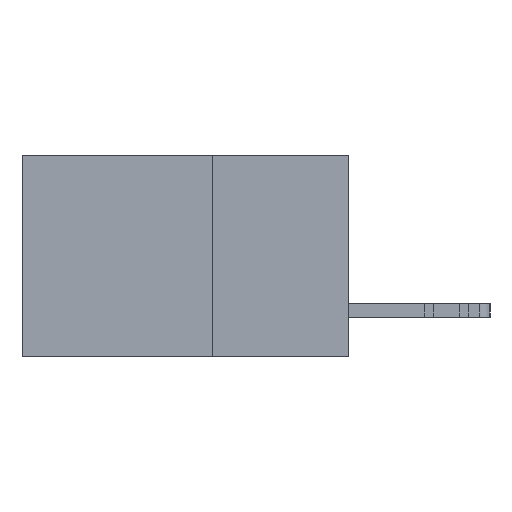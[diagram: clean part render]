
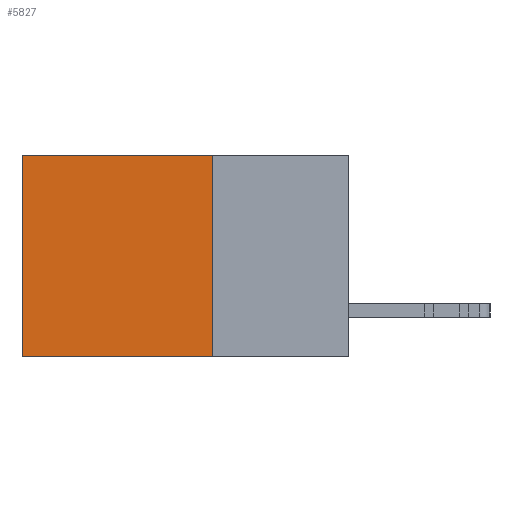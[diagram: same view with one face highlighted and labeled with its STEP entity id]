
A CAD part, left-side view. The second image highlights one B-rep face of the part: STEP entity #5827.
In plain terms, the highlighted planar face has unit normal (-1, 0, 0).
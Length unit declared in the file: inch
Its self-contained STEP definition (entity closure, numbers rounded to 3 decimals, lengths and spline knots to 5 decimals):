
#267 = DIRECTION ( 'NONE',  ( 1., 0., 0. ) ) ;
#484 = VERTEX_POINT ( 'NONE', #6605 ) ;
#1245 = CARTESIAN_POINT ( 'NONE',  ( 0.298, 0.25, -0.37 ) ) ;
#1613 = DIRECTION ( 'NONE',  ( 0., 0., -1. ) ) ;
#3563 = LINE ( 'NONE', #21621, #25673 ) ;
#3666 = EDGE_CURVE ( 'NONE', #4338, #14736, #26336, .T. ) ;
#3944 = DIRECTION ( 'NONE',  ( 0., 0., -1. ) ) ;
#4338 = VERTEX_POINT ( 'NONE', #23929 ) ;
#4529 = VECTOR ( 'NONE', #13940, 39.37008 ) ;
#5827 = ADVANCED_FACE ( 'NONE', ( #6676 ), #24602, .F. ) ;
#6118 = EDGE_CURVE ( 'NONE', #14736, #484, #27677, .T. ) ;
#6283 = EDGE_CURVE ( 'NONE', #4338, #20408, #28006, .T. ) ;
#6605 = CARTESIAN_POINT ( 'NONE',  ( 0.298, 0.6, -0.37 ) ) ;
#6676 = FACE_OUTER_BOUND ( 'NONE', #10706, .T. ) ;
#6752 = CARTESIAN_POINT ( 'NONE',  ( 0.298, 0.25, 0. ) ) ;
#10082 = ORIENTED_EDGE ( 'NONE', *, *, #6118, .F. ) ;
#10706 = EDGE_LOOP ( 'NONE', ( #10852, #10082, #19434, #26820 ) ) ;
#10852 = ORIENTED_EDGE ( 'NONE', *, *, #11824, .T. ) ;
#11417 = CARTESIAN_POINT ( 'NONE',  ( 0.298, 0.25, 0. ) ) ;
#11824 = EDGE_CURVE ( 'NONE', #20408, #484, #3563, .T. ) ;
#13940 = DIRECTION ( 'NONE',  ( 0., 1., 0. ) ) ;
#14221 = CARTESIAN_POINT ( 'NONE',  ( 0.298, 0.6, 0. ) ) ;
#14736 = VERTEX_POINT ( 'NONE', #19982 ) ;
#15842 = DIRECTION ( 'NONE',  ( 0., 0., -1. ) ) ;
#16034 = VECTOR ( 'NONE', #3944, 39.37008 ) ;
#16340 = AXIS2_PLACEMENT_3D ( 'NONE', #11417, #267, #15842 ) ;
#19434 = ORIENTED_EDGE ( 'NONE', *, *, #3666, .F. ) ;
#19982 = CARTESIAN_POINT ( 'NONE',  ( 0.298, 0.25, -0.37 ) ) ;
#20408 = VERTEX_POINT ( 'NONE', #14221 ) ;
#21621 = CARTESIAN_POINT ( 'NONE',  ( 0.298, 0.6, 0. ) ) ;
#23861 = CARTESIAN_POINT ( 'NONE',  ( 0.298, 0.25, 0. ) ) ;
#23929 = CARTESIAN_POINT ( 'NONE',  ( 0.298, 0.25, 0. ) ) ;
#24602 = PLANE ( 'NONE',  #16340 ) ;
#25649 = DIRECTION ( 'NONE',  ( 0., 1., 0. ) ) ;
#25673 = VECTOR ( 'NONE', #1613, 39.37008 ) ;
#26298 = VECTOR ( 'NONE', #25649, 39.37008 ) ;
#26336 = LINE ( 'NONE', #23861, #16034 ) ;
#26820 = ORIENTED_EDGE ( 'NONE', *, *, #6283, .T. ) ;
#27677 = LINE ( 'NONE', #1245, #26298 ) ;
#28006 = LINE ( 'NONE', #6752, #4529 ) ;
